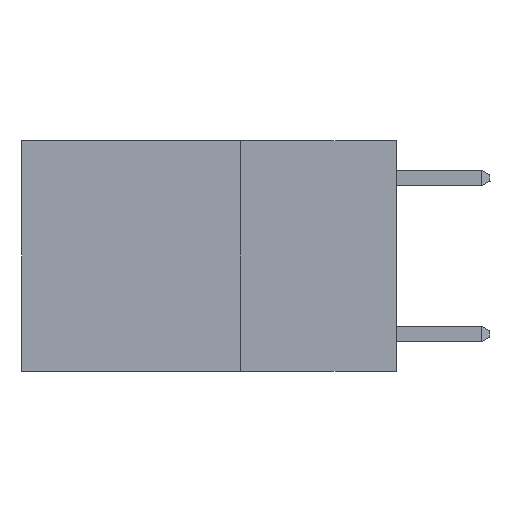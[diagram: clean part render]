
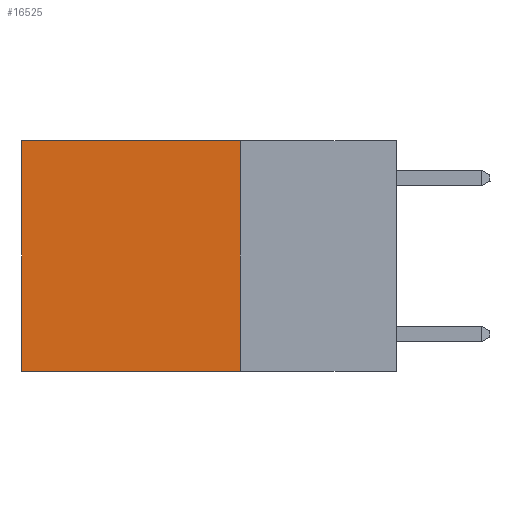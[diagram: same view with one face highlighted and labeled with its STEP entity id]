
A CAD part, left-side view. The second image highlights one B-rep face of the part: STEP entity #16525.
In plain terms, the highlighted planar face has unit normal (-1, 0, 0).
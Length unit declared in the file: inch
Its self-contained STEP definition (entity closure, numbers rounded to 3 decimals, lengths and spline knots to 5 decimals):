
#1030 = EDGE_LOOP ( 'NONE', ( #22331, #26884, #27596, #19242 ) ) ;
#4836 = DIRECTION ( 'NONE',  ( 0., 1., 0. ) ) ;
#5743 = VERTEX_POINT ( 'NONE', #17382 ) ;
#6117 = EDGE_CURVE ( 'NONE', #7088, #21532, #17453, .T. ) ;
#6832 = CARTESIAN_POINT ( 'NONE',  ( 0.2625, 0.6, 0. ) ) ;
#7088 = VERTEX_POINT ( 'NONE', #28920 ) ;
#7440 = DIRECTION ( 'NONE',  ( 0., 0., -1. ) ) ;
#8214 = DIRECTION ( 'NONE',  ( 0., 0., -1. ) ) ;
#9275 = VERTEX_POINT ( 'NONE', #12224 ) ;
#9294 = LINE ( 'NONE', #6832, #10532 ) ;
#9717 = CARTESIAN_POINT ( 'NONE',  ( 0.2625, 0.25, 0. ) ) ;
#10532 = VECTOR ( 'NONE', #7440, 39.37008 ) ;
#12224 = CARTESIAN_POINT ( 'NONE',  ( 0.2625, 0.25, 0. ) ) ;
#12362 = CARTESIAN_POINT ( 'NONE',  ( 0.2625, 0.25, 0. ) ) ;
#12512 = LINE ( 'NONE', #12362, #22804 ) ;
#16525 = ADVANCED_FACE ( 'NONE', ( #20199 ), #19904, .F. ) ;
#17157 = DIRECTION ( 'NONE',  ( 0., 1., 0. ) ) ;
#17382 = CARTESIAN_POINT ( 'NONE',  ( 0.2625, 0.6, 0. ) ) ;
#17453 = LINE ( 'NONE', #22055, #26968 ) ;
#19114 = DIRECTION ( 'NONE',  ( 0., 0., -1. ) ) ;
#19242 = ORIENTED_EDGE ( 'NONE', *, *, #26436, .T. ) ;
#19904 = PLANE ( 'NONE',  #27807 ) ;
#20199 = FACE_OUTER_BOUND ( 'NONE', #1030, .T. ) ;
#21253 = LINE ( 'NONE', #9717, #28775 ) ;
#21532 = VERTEX_POINT ( 'NONE', #24537 ) ;
#22055 = CARTESIAN_POINT ( 'NONE',  ( 0.2625, 0.25, -0.37 ) ) ;
#22331 = ORIENTED_EDGE ( 'NONE', *, *, #24913, .T. ) ;
#22665 = CARTESIAN_POINT ( 'NONE',  ( 0.2625, 0.25, 0. ) ) ;
#22804 = VECTOR ( 'NONE', #17157, 39.37008 ) ;
#24537 = CARTESIAN_POINT ( 'NONE',  ( 0.2625, 0.6, -0.37 ) ) ;
#24913 = EDGE_CURVE ( 'NONE', #5743, #21532, #9294, .T. ) ;
#26436 = EDGE_CURVE ( 'NONE', #9275, #5743, #12512, .T. ) ;
#26734 = EDGE_CURVE ( 'NONE', #9275, #7088, #21253, .T. ) ;
#26884 = ORIENTED_EDGE ( 'NONE', *, *, #6117, .F. ) ;
#26968 = VECTOR ( 'NONE', #4836, 39.37008 ) ;
#27596 = ORIENTED_EDGE ( 'NONE', *, *, #26734, .F. ) ;
#27807 = AXIS2_PLACEMENT_3D ( 'NONE', #22665, #29305, #8214 ) ;
#28775 = VECTOR ( 'NONE', #19114, 39.37008 ) ;
#28920 = CARTESIAN_POINT ( 'NONE',  ( 0.2625, 0.25, -0.37 ) ) ;
#29305 = DIRECTION ( 'NONE',  ( 1., 0., 0. ) ) ;
